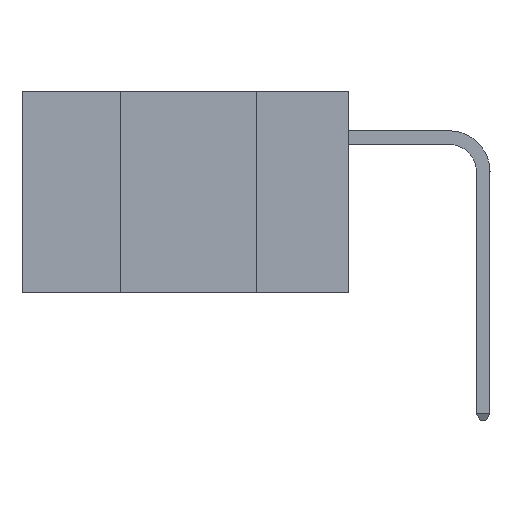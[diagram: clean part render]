
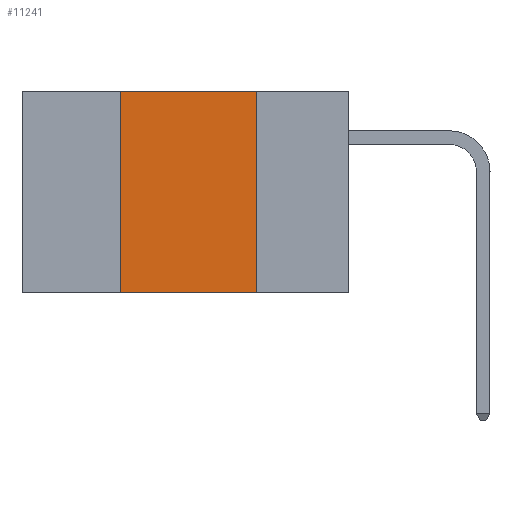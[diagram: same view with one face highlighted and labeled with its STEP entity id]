
A CAD part, left-side view. The second image highlights one B-rep face of the part: STEP entity #11241.
In plain terms, the highlighted planar face has unit normal (-1, 0, 0).
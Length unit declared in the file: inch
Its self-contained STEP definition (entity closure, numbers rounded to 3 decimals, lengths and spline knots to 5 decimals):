
#710 = CARTESIAN_POINT ( 'NONE',  ( 0., 0.6, 0. ) ) ;
#805 = DIRECTION ( 'NONE',  ( 0., -1., 0. ) ) ;
#2446 = PLANE ( 'NONE',  #27531 ) ;
#2682 = VECTOR ( 'NONE', #10785, 39.37008 ) ;
#2897 = ORIENTED_EDGE ( 'NONE', *, *, #23304, .F. ) ;
#4165 = VECTOR ( 'NONE', #10859, 39.37008 ) ;
#4738 = DIRECTION ( 'NONE',  ( 0., 0., -1. ) ) ;
#4851 = VERTEX_POINT ( 'NONE', #17662 ) ;
#5984 = LINE ( 'NONE', #13724, #17454 ) ;
#6055 = VECTOR ( 'NONE', #805, 39.37008 ) ;
#6381 = EDGE_CURVE ( 'NONE', #22560, #24177, #5984, .T. ) ;
#10115 = EDGE_CURVE ( 'NONE', #4851, #22560, #12213, .T. ) ;
#10785 = DIRECTION ( 'NONE',  ( 0., -1., 0. ) ) ;
#10859 = DIRECTION ( 'NONE',  ( 0., 0., 1. ) ) ;
#11241 = ADVANCED_FACE ( 'NONE', ( #12841 ), #2446, .F. ) ;
#11861 = CARTESIAN_POINT ( 'NONE',  ( 0., 0.17, 0. ) ) ;
#12087 = EDGE_LOOP ( 'NONE', ( #20323, #17694, #2897, #19884 ) ) ;
#12213 = LINE ( 'NONE', #710, #6055 ) ;
#12841 = FACE_OUTER_BOUND ( 'NONE', #12087, .T. ) ;
#13724 = CARTESIAN_POINT ( 'NONE',  ( 0., 0.17, 0. ) ) ;
#13886 = CARTESIAN_POINT ( 'NONE',  ( 0., 0.6, 0. ) ) ;
#14014 = CARTESIAN_POINT ( 'NONE',  ( 0., 0.17, -0.37 ) ) ;
#14163 = CARTESIAN_POINT ( 'NONE',  ( 0., 0.42, -0.37 ) ) ;
#15991 = DIRECTION ( 'NONE',  ( 0., 0., -1. ) ) ;
#17454 = VECTOR ( 'NONE', #15991, 39.37008 ) ;
#17630 = CARTESIAN_POINT ( 'NONE',  ( 0., 0.42, 0. ) ) ;
#17662 = CARTESIAN_POINT ( 'NONE',  ( 0., 0.42, 0. ) ) ;
#17694 = ORIENTED_EDGE ( 'NONE', *, *, #10115, .F. ) ;
#18457 = DIRECTION ( 'NONE',  ( 1., 0., 0. ) ) ;
#19884 = ORIENTED_EDGE ( 'NONE', *, *, #24556, .T. ) ;
#20323 = ORIENTED_EDGE ( 'NONE', *, *, #6381, .F. ) ;
#22560 = VERTEX_POINT ( 'NONE', #11861 ) ;
#23011 = LINE ( 'NONE', #17630, #4165 ) ;
#23304 = EDGE_CURVE ( 'NONE', #25368, #4851, #23011, .T. ) ;
#24177 = VERTEX_POINT ( 'NONE', #14014 ) ;
#24556 = EDGE_CURVE ( 'NONE', #25368, #24177, #26754, .T. ) ;
#25368 = VERTEX_POINT ( 'NONE', #14163 ) ;
#26503 = CARTESIAN_POINT ( 'NONE',  ( 0., 0.6, -0.37 ) ) ;
#26754 = LINE ( 'NONE', #26503, #2682 ) ;
#27531 = AXIS2_PLACEMENT_3D ( 'NONE', #13886, #18457, #4738 ) ;
